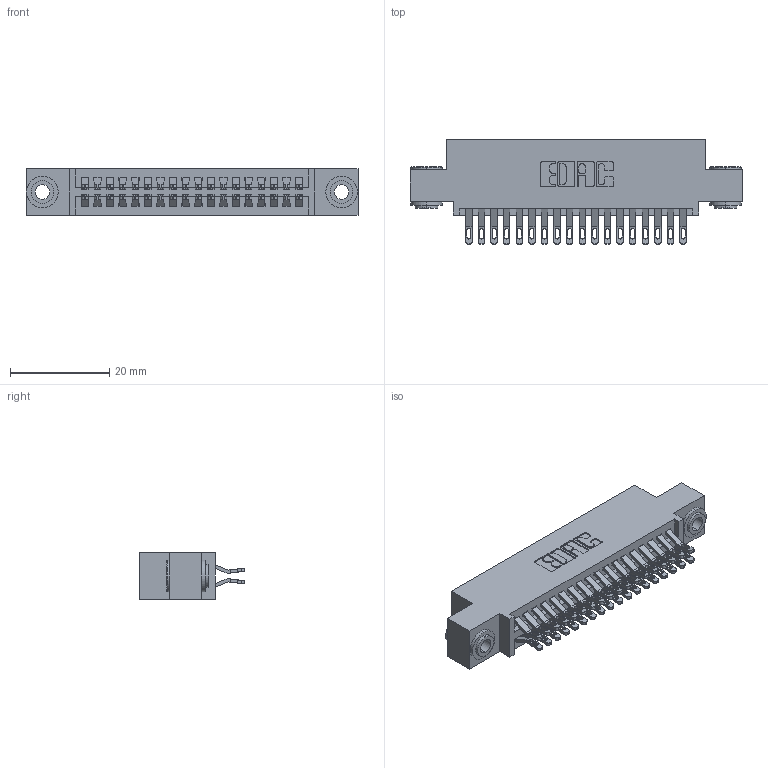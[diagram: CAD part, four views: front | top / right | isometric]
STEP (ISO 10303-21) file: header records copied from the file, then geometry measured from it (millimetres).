
FILE_DESCRIPTION (( 'STEP AP203' ), '1' );
FILE_NAME ('345-036-555-503.STEP', '2019-10-28T12:36:39', ( '' ), ( '' ), 'SwSTEP 2.0', 'SolidWorks 2016', '' );
FILE_SCHEMA (( 'CONFIG_CONTROL_DESIGN' ));
Length unit declared in the file: inch
Products named in the file (4): 345-036-555-503; 345 Part_0.110 Offset - 0.156 Dia-TH; 345-250-002_345-250-002-102; 345-292-001_555 Tail
Assembly tree (39 placements, depth 2):
  345-036-555-503
    345 Part_0.110 Offset - 0.156 Dia-TH
    345-292-001_555 Tail  x36
    345-250-002_345-250-002-102  x2
Bounding box: 66.93 x 21.13 x 9.4 mm (x, y, z)
Volume: 6329.2 mm3; surface area: 9551.7 mm2
Topology: 39 solids, 39 shells, 2184 faces, 6801 edges, 4530 vertices
Faces by surface type: plane 1210, cylinder 966, cone 8
Entity records: 18462 total; most frequent: CARTESIAN_POINT 3129, ORIENTED_EDGE 3026, DIRECTION 2787, EDGE_CURVE 1513, LINE 1265, VECTOR 1265, VERTEX_POINT 1006, AXIS2_PLACEMENT_3D 761
